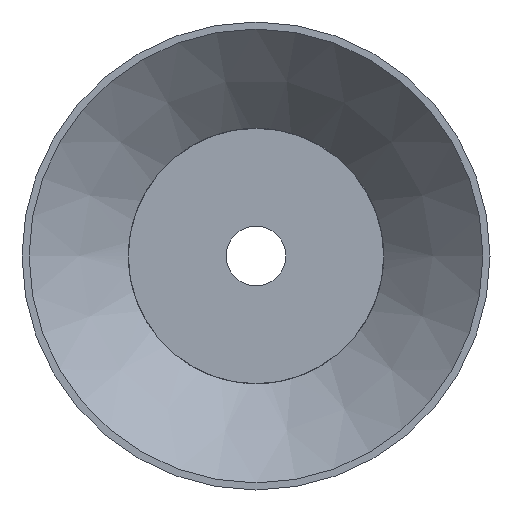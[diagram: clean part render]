
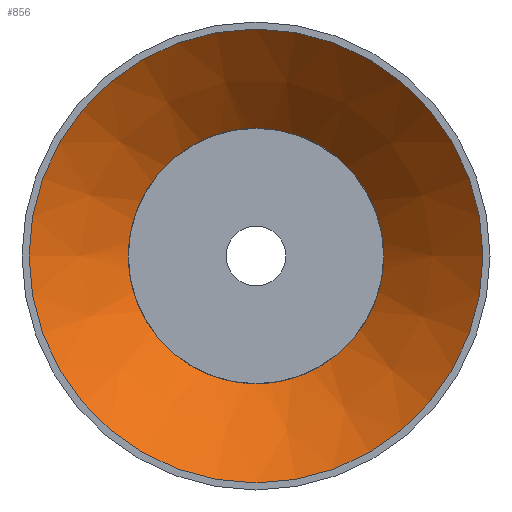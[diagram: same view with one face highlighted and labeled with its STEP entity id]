
A CAD part, front view. The second image highlights one B-rep face of the part: STEP entity #856.
In plain terms, the highlighted conical face has half-angle 45.227 degrees and reference radius 31.679 mm.
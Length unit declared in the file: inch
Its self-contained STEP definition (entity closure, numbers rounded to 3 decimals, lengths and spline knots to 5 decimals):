
#118=(
BOUNDED_CURVE()
B_SPLINE_CURVE(2,(#1179,#1180,#1181),.UNSPECIFIED.,.F.,.F.)
B_SPLINE_CURVE_WITH_KNOTS((3,3),(0.,0.0223),.UNSPECIFIED.)
CURVE()
GEOMETRIC_REPRESENTATION_ITEM()
RATIONAL_B_SPLINE_CURVE((1.,1.,1.))
REPRESENTATION_ITEM('')
);
#119=(
BOUNDED_CURVE()
B_SPLINE_CURVE(2,(#1185,#1186,#1187),.UNSPECIFIED.,.F.,.F.)
B_SPLINE_CURVE_WITH_KNOTS((3,3),(0.7967,0.819),
 .UNSPECIFIED.)
CURVE()
GEOMETRIC_REPRESENTATION_ITEM()
RATIONAL_B_SPLINE_CURVE((1.,1.,1.))
REPRESENTATION_ITEM('')
);
#120=(
BOUNDED_CURVE()
B_SPLINE_CURVE(2,(#1190,#1191,#1192),.UNSPECIFIED.,.F.,.F.)
B_SPLINE_CURVE_WITH_KNOTS((3,3),(0.,0.0223),.UNSPECIFIED.)
CURVE()
GEOMETRIC_REPRESENTATION_ITEM()
RATIONAL_B_SPLINE_CURVE((1.,1.,1.))
REPRESENTATION_ITEM('')
);
#121=(
BOUNDED_CURVE()
B_SPLINE_CURVE(2,(#1194,#1195,#1196),.UNSPECIFIED.,.F.,.F.)
B_SPLINE_CURVE_WITH_KNOTS((3,3),(0.79696,0.81926),
 .UNSPECIFIED.)
CURVE()
GEOMETRIC_REPRESENTATION_ITEM()
RATIONAL_B_SPLINE_CURVE((1.,1.,1.))
REPRESENTATION_ITEM('')
);
#122=(
BOUNDED_CURVE()
B_SPLINE_CURVE(2,(#1199,#1200,#1201),.UNSPECIFIED.,.F.,.F.)
B_SPLINE_CURVE_WITH_KNOTS((3,3),(0.,0.0223),.UNSPECIFIED.)
CURVE()
GEOMETRIC_REPRESENTATION_ITEM()
RATIONAL_B_SPLINE_CURVE((1.,1.,1.))
REPRESENTATION_ITEM('')
);
#123=(
BOUNDED_CURVE()
B_SPLINE_CURVE(2,(#1203,#1204,#1205),.UNSPECIFIED.,.F.,.F.)
B_SPLINE_CURVE_WITH_KNOTS((3,3),(0.79657,0.81887),
 .UNSPECIFIED.)
CURVE()
GEOMETRIC_REPRESENTATION_ITEM()
RATIONAL_B_SPLINE_CURVE((1.,1.,1.))
REPRESENTATION_ITEM('')
);
#124=(
BOUNDED_CURVE()
B_SPLINE_CURVE(2,(#1208,#1209,#1210),.UNSPECIFIED.,.F.,.F.)
B_SPLINE_CURVE_WITH_KNOTS((3,3),(0.,0.0223),.UNSPECIFIED.)
CURVE()
GEOMETRIC_REPRESENTATION_ITEM()
RATIONAL_B_SPLINE_CURVE((1.,1.,1.))
REPRESENTATION_ITEM('')
);
#125=(
BOUNDED_CURVE()
B_SPLINE_CURVE(2,(#1212,#1213,#1214),.UNSPECIFIED.,.F.,.F.)
B_SPLINE_CURVE_WITH_KNOTS((3,3),(0.79673,0.81903),
 .UNSPECIFIED.)
CURVE()
GEOMETRIC_REPRESENTATION_ITEM()
RATIONAL_B_SPLINE_CURVE((1.,1.,1.))
REPRESENTATION_ITEM('')
);
#127=CONICAL_SURFACE('',#922,1.24722,0.789);
#134=FACE_OUTER_BOUND('',#174,.T.);
#174=EDGE_LOOP('',(#575,#576,#577,#578,#579,#580,#581,#582,#583,#584,#585,
#586,#587,#588,#589,#590,#591,#592,#593,#594,#595));
#220=LINE('',#1175,#250);
#250=VECTOR('',#1016,1.24722);
#279=CIRCLE('',#915,0.89444);
#281=CIRCLE('',#918,0.89444);
#282=CIRCLE('',#920,0.89444);
#284=CIRCLE('',#923,1.6);
#285=CIRCLE('',#924,0.9);
#286=CIRCLE('',#925,0.89444);
#287=CIRCLE('',#926,0.9);
#288=CIRCLE('',#927,0.9);
#289=CIRCLE('',#928,0.9);
#290=CIRCLE('',#929,0.9);
#291=CIRCLE('',#930,1.6);
#315=VERTEX_POINT('',#1145);
#317=VERTEX_POINT('',#1149);
#319=VERTEX_POINT('',#1154);
#321=VERTEX_POINT('',#1158);
#322=VERTEX_POINT('',#1162);
#324=VERTEX_POINT('',#1165);
#326=VERTEX_POINT('',#1171);
#327=VERTEX_POINT('',#1172);
#328=VERTEX_POINT('',#1174);
#329=VERTEX_POINT('',#1176);
#330=VERTEX_POINT('',#1178);
#331=VERTEX_POINT('',#1182);
#332=VERTEX_POINT('',#1184);
#333=VERTEX_POINT('',#1188);
#334=VERTEX_POINT('',#1193);
#335=VERTEX_POINT('',#1197);
#336=VERTEX_POINT('',#1202);
#337=VERTEX_POINT('',#1206);
#338=VERTEX_POINT('',#1211);
#419=EDGE_CURVE('',#317,#315,#279,.T.);
#423=EDGE_CURVE('',#321,#319,#281,.T.);
#425=EDGE_CURVE('',#322,#324,#282,.T.);
#428=EDGE_CURVE('',#326,#327,#284,.T.);
#429=EDGE_CURVE('',#327,#328,#220,.T.);
#430=EDGE_CURVE('',#329,#328,#285,.T.);
#431=EDGE_CURVE('',#330,#329,#118,.T.);
#432=EDGE_CURVE('',#331,#330,#286,.T.);
#433=EDGE_CURVE('',#332,#331,#119,.T.);
#434=EDGE_CURVE('',#333,#332,#287,.T.);
#435=EDGE_CURVE('',#319,#333,#120,.T.);
#436=EDGE_CURVE('',#334,#321,#121,.T.);
#437=EDGE_CURVE('',#335,#334,#288,.T.);
#438=EDGE_CURVE('',#315,#335,#122,.T.);
#439=EDGE_CURVE('',#336,#317,#123,.T.);
#440=EDGE_CURVE('',#337,#336,#289,.T.);
#441=EDGE_CURVE('',#324,#337,#124,.T.);
#442=EDGE_CURVE('',#338,#322,#125,.T.);
#443=EDGE_CURVE('',#328,#338,#290,.T.);
#444=EDGE_CURVE('',#327,#326,#291,.T.);
#575=ORIENTED_EDGE('',*,*,#428,.T.);
#576=ORIENTED_EDGE('',*,*,#429,.T.);
#577=ORIENTED_EDGE('',*,*,#430,.F.);
#578=ORIENTED_EDGE('',*,*,#431,.F.);
#579=ORIENTED_EDGE('',*,*,#432,.F.);
#580=ORIENTED_EDGE('',*,*,#433,.F.);
#581=ORIENTED_EDGE('',*,*,#434,.F.);
#582=ORIENTED_EDGE('',*,*,#435,.F.);
#583=ORIENTED_EDGE('',*,*,#423,.F.);
#584=ORIENTED_EDGE('',*,*,#436,.F.);
#585=ORIENTED_EDGE('',*,*,#437,.F.);
#586=ORIENTED_EDGE('',*,*,#438,.F.);
#587=ORIENTED_EDGE('',*,*,#419,.F.);
#588=ORIENTED_EDGE('',*,*,#439,.F.);
#589=ORIENTED_EDGE('',*,*,#440,.F.);
#590=ORIENTED_EDGE('',*,*,#441,.F.);
#591=ORIENTED_EDGE('',*,*,#425,.F.);
#592=ORIENTED_EDGE('',*,*,#442,.F.);
#593=ORIENTED_EDGE('',*,*,#443,.F.);
#594=ORIENTED_EDGE('',*,*,#429,.F.);
#595=ORIENTED_EDGE('',*,*,#444,.T.);
#856=ADVANCED_FACE('',(#134),#127,.F.);
#915=AXIS2_PLACEMENT_3D('',#1151,#994,#995);
#918=AXIS2_PLACEMENT_3D('',#1160,#1002,#1003);
#920=AXIS2_PLACEMENT_3D('',#1166,#1007,#1008);
#922=AXIS2_PLACEMENT_3D('',#1170,#1012,#1013);
#923=AXIS2_PLACEMENT_3D('',#1173,#1014,#1015);
#924=AXIS2_PLACEMENT_3D('',#1177,#1017,#1018);
#925=AXIS2_PLACEMENT_3D('',#1183,#1019,#1020);
#926=AXIS2_PLACEMENT_3D('',#1189,#1021,#1022);
#927=AXIS2_PLACEMENT_3D('',#1198,#1023,#1024);
#928=AXIS2_PLACEMENT_3D('',#1207,#1025,#1026);
#929=AXIS2_PLACEMENT_3D('',#1215,#1027,#1028);
#930=AXIS2_PLACEMENT_3D('',#1216,#1029,#1030);
#994=DIRECTION('center_axis',(0.,-1.,0.));
#995=DIRECTION('ref_axis',(1.,0.,0.));
#1002=DIRECTION('center_axis',(0.,-1.,0.));
#1003=DIRECTION('ref_axis',(1.,0.,0.));
#1007=DIRECTION('center_axis',(0.,-1.,0.));
#1008=DIRECTION('ref_axis',(1.,0.,0.));
#1012=DIRECTION('center_axis',(0.,-1.,0.));
#1013=DIRECTION('ref_axis',(1.,0.,0.));
#1014=DIRECTION('center_axis',(0.,-1.,0.));
#1015=DIRECTION('ref_axis',(1.,0.,0.));
#1016=DIRECTION('',(0.71,0.704,0.));
#1017=DIRECTION('center_axis',(0.,-1.,0.));
#1018=DIRECTION('ref_axis',(1.,0.,0.));
#1019=DIRECTION('center_axis',(0.,-1.,0.));
#1020=DIRECTION('ref_axis',(1.,0.,0.));
#1021=DIRECTION('center_axis',(0.,-1.,0.));
#1022=DIRECTION('ref_axis',(1.,0.,0.));
#1023=DIRECTION('center_axis',(0.,-1.,0.));
#1024=DIRECTION('ref_axis',(1.,0.,0.));
#1025=DIRECTION('center_axis',(0.,-1.,0.));
#1026=DIRECTION('ref_axis',(1.,0.,0.));
#1027=DIRECTION('center_axis',(0.,-1.,0.));
#1028=DIRECTION('ref_axis',(1.,0.,0.));
#1029=DIRECTION('center_axis',(0.,-1.,0.));
#1030=DIRECTION('ref_axis',(1.,0.,0.));
#1145=CARTESIAN_POINT('',(0.88883,0.7,-0.09999));
#1149=CARTESIAN_POINT('',(0.10011,0.7,-0.88882));
#1151=CARTESIAN_POINT('Origin',(0.,0.7,0.));
#1154=CARTESIAN_POINT('',(0.09981,0.7,0.88886));
#1158=CARTESIAN_POINT('',(0.88885,0.7,0.09988));
#1160=CARTESIAN_POINT('Origin',(0.,0.7,0.));
#1162=CARTESIAN_POINT('',(-0.88883,0.7,-0.10001));
#1165=CARTESIAN_POINT('',(-0.09999,0.7,-0.88883));
#1166=CARTESIAN_POINT('Origin',(0.,0.7,0.));
#1170=CARTESIAN_POINT('Origin',(0.,0.35,0.));
#1171=CARTESIAN_POINT('',(1.6,0.,0.));
#1172=CARTESIAN_POINT('',(-1.6,0.,0.));
#1173=CARTESIAN_POINT('Origin',(0.,0.,0.));
#1174=CARTESIAN_POINT('',(-0.9,0.69448,0.));
#1175=CARTESIAN_POINT('',(-1.24722,0.35,0.));
#1176=CARTESIAN_POINT('',(-0.89443,0.69448,0.10001));
#1177=CARTESIAN_POINT('Origin',(0.,0.69448,0.));
#1178=CARTESIAN_POINT('',(-0.88883,0.7,0.10001));
#1179=CARTESIAN_POINT('Ctrl Pts',(-0.88883,0.7,
0.10001));
#1180=CARTESIAN_POINT('Ctrl Pts',(-0.89162,0.69725,
0.10001));
#1181=CARTESIAN_POINT('Ctrl Pts',(-0.89443,0.69448,
0.10001));
#1182=CARTESIAN_POINT('',(-0.10002,0.7,0.88883));
#1183=CARTESIAN_POINT('Origin',(0.,0.7,0.));
#1184=CARTESIAN_POINT('',(-0.10003,0.69448,0.89442));
#1185=CARTESIAN_POINT('Ctrl Pts',(-0.10003,0.69448,
0.89442));
#1186=CARTESIAN_POINT('Ctrl Pts',(-0.10002,0.69725,
0.89162));
#1187=CARTESIAN_POINT('Ctrl Pts',(-0.10002,0.7,
0.88883));
#1188=CARTESIAN_POINT('',(0.0998,0.69448,0.89445));
#1189=CARTESIAN_POINT('Origin',(0.,0.69448,0.));
#1190=CARTESIAN_POINT('Ctrl Pts',(0.09981,0.7,
0.88886));
#1191=CARTESIAN_POINT('Ctrl Pts',(0.0998,0.69725,
0.89164));
#1192=CARTESIAN_POINT('Ctrl Pts',(0.0998,0.69448,
0.89445));
#1193=CARTESIAN_POINT('',(0.89444,0.69448,0.09987));
#1194=CARTESIAN_POINT('Ctrl Pts',(0.89444,0.69448,0.09987));
#1195=CARTESIAN_POINT('Ctrl Pts',(0.89164,0.69725,0.09988));
#1196=CARTESIAN_POINT('Ctrl Pts',(0.88885,0.7,0.09988));
#1197=CARTESIAN_POINT('',(0.89443,0.69448,-0.09999));
#1198=CARTESIAN_POINT('Origin',(0.,0.69448,0.));
#1199=CARTESIAN_POINT('Ctrl Pts',(0.88883,0.7,-0.09999));
#1200=CARTESIAN_POINT('Ctrl Pts',(0.89162,0.69725,-0.09999));
#1201=CARTESIAN_POINT('Ctrl Pts',(0.89443,0.69448,-0.09999));
#1202=CARTESIAN_POINT('',(0.10011,0.69448,-0.89441));
#1203=CARTESIAN_POINT('Ctrl Pts',(0.10011,0.69448,-0.89441));
#1204=CARTESIAN_POINT('Ctrl Pts',(0.10011,0.69725,-0.89161));
#1205=CARTESIAN_POINT('Ctrl Pts',(0.10011,0.7,-0.88882));
#1206=CARTESIAN_POINT('',(-0.09999,0.69448,-0.89443));
#1207=CARTESIAN_POINT('Origin',(0.,0.69448,0.));
#1208=CARTESIAN_POINT('Ctrl Pts',(-0.09999,0.7,
-0.88883));
#1209=CARTESIAN_POINT('Ctrl Pts',(-0.09999,0.69725,
-0.89162));
#1210=CARTESIAN_POINT('Ctrl Pts',(-0.09999,0.69448,
-0.89443));
#1211=CARTESIAN_POINT('',(-0.89443,0.69448,-0.10001));
#1212=CARTESIAN_POINT('Ctrl Pts',(-0.89443,0.69448,
-0.10001));
#1213=CARTESIAN_POINT('Ctrl Pts',(-0.89162,0.69725,
-0.10001));
#1214=CARTESIAN_POINT('Ctrl Pts',(-0.88883,0.7,
-0.10001));
#1215=CARTESIAN_POINT('Origin',(0.,0.69448,0.));
#1216=CARTESIAN_POINT('Origin',(0.,0.,0.));
